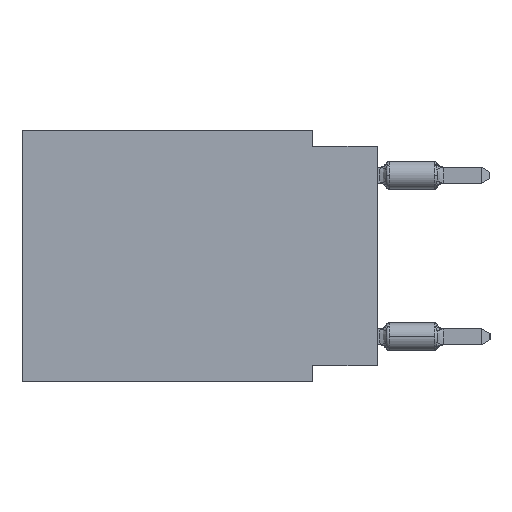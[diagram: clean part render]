
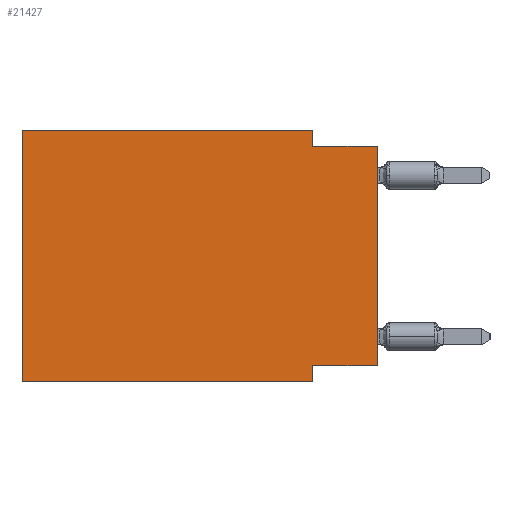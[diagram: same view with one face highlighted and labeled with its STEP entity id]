
A CAD part, left-side view. The second image highlights one B-rep face of the part: STEP entity #21427.
In plain terms, the highlighted planar face has unit normal (-1, 0, 0).
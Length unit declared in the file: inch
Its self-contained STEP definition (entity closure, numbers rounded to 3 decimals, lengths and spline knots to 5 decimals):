
#96 = CARTESIAN_POINT ( 'NONE',  ( 0., 0.55, 0. ) ) ;
#1198 = CARTESIAN_POINT ( 'NONE',  ( 0., 0.1, 0. ) ) ;
#1416 = DIRECTION ( 'NONE',  ( 0., 0., -1. ) ) ;
#1516 = EDGE_LOOP ( 'NONE', ( #18614, #11965, #40280, #30509, #34123, #24279, #11239, #11448 ) ) ;
#1558 = CARTESIAN_POINT ( 'NONE',  ( 0., 0.1, 0. ) ) ;
#2516 = EDGE_CURVE ( 'NONE', #9751, #14857, #4752, .T. ) ;
#2631 = EDGE_CURVE ( 'NONE', #19901, #14253, #5404, .T. ) ;
#2844 = VECTOR ( 'NONE', #1416, 39.37008 ) ;
#4245 = VERTEX_POINT ( 'NONE', #96 ) ;
#4752 = LINE ( 'NONE', #18272, #2844 ) ;
#5187 = VECTOR ( 'NONE', #41019, 39.37008 ) ;
#5231 = CARTESIAN_POINT ( 'NONE',  ( 0., 0.55, -0.39 ) ) ;
#5404 = LINE ( 'NONE', #19139, #32566 ) ;
#5408 = LINE ( 'NONE', #1198, #36933 ) ;
#8339 = DIRECTION ( 'NONE',  ( 0., -1., 0. ) ) ;
#9701 = CARTESIAN_POINT ( 'NONE',  ( 0., 0.1, -0.39 ) ) ;
#9704 = DIRECTION ( 'NONE',  ( 0., 1., 0. ) ) ;
#9751 = VERTEX_POINT ( 'NONE', #39318 ) ;
#9925 = CARTESIAN_POINT ( 'NONE',  ( 0., 0., -0.365 ) ) ;
#11239 = ORIENTED_EDGE ( 'NONE', *, *, #2516, .F. ) ;
#11354 = FACE_OUTER_BOUND ( 'NONE', #1516, .T. ) ;
#11448 = ORIENTED_EDGE ( 'NONE', *, *, #34178, .F. ) ;
#11965 = ORIENTED_EDGE ( 'NONE', *, *, #37853, .F. ) ;
#12773 = DIRECTION ( 'NONE',  ( 0., -1., 0. ) ) ;
#12815 = DIRECTION ( 'NONE',  ( 0., 0., -1. ) ) ;
#13987 = LINE ( 'NONE', #24176, #5187 ) ;
#14253 = VERTEX_POINT ( 'NONE', #35989 ) ;
#14857 = VERTEX_POINT ( 'NONE', #9701 ) ;
#17372 = VERTEX_POINT ( 'NONE', #1558 ) ;
#18272 = CARTESIAN_POINT ( 'NONE',  ( 0., 0.1, -0.39 ) ) ;
#18494 = DIRECTION ( 'NONE',  ( 0., 0., -1. ) ) ;
#18614 = ORIENTED_EDGE ( 'NONE', *, *, #2631, .T. ) ;
#18812 = CARTESIAN_POINT ( 'NONE',  ( 0., 0.55, 0. ) ) ;
#19139 = CARTESIAN_POINT ( 'NONE',  ( 0., 0., 0. ) ) ;
#19901 = VERTEX_POINT ( 'NONE', #39906 ) ;
#20064 = LINE ( 'NONE', #43772, #32785 ) ;
#20338 = VECTOR ( 'NONE', #9704, 39.37008 ) ;
#21427 = ADVANCED_FACE ( 'NONE', ( #11354 ), #26325, .F. ) ;
#24176 = CARTESIAN_POINT ( 'NONE',  ( 0., 0.55, 0. ) ) ;
#24279 = ORIENTED_EDGE ( 'NONE', *, *, #38174, .T. ) ;
#26143 = DIRECTION ( 'NONE',  ( 0., -1., 0. ) ) ;
#26325 = PLANE ( 'NONE',  #37262 ) ;
#30509 = ORIENTED_EDGE ( 'NONE', *, *, #43373, .F. ) ;
#30599 = VERTEX_POINT ( 'NONE', #30624 ) ;
#30624 = CARTESIAN_POINT ( 'NONE',  ( 0., 0.55, -0.39 ) ) ;
#31096 = EDGE_CURVE ( 'NONE', #30599, #4245, #13987, .T. ) ;
#32556 = DIRECTION ( 'NONE',  ( 1., 0., 0. ) ) ;
#32566 = VECTOR ( 'NONE', #43281, 39.37008 ) ;
#32785 = VECTOR ( 'NONE', #12773, 39.37008 ) ;
#33382 = VERTEX_POINT ( 'NONE', #33735 ) ;
#33735 = CARTESIAN_POINT ( 'NONE',  ( 0., 0.1, -0.025 ) ) ;
#34123 = ORIENTED_EDGE ( 'NONE', *, *, #31096, .F. ) ;
#34178 = EDGE_CURVE ( 'NONE', #19901, #9751, #40501, .T. ) ;
#35989 = CARTESIAN_POINT ( 'NONE',  ( 0., 0., -0.025 ) ) ;
#36933 = VECTOR ( 'NONE', #18494, 39.37008 ) ;
#37262 = AXIS2_PLACEMENT_3D ( 'NONE', #18812, #32556, #12815 ) ;
#37853 = EDGE_CURVE ( 'NONE', #33382, #14253, #42783, .T. ) ;
#38174 = EDGE_CURVE ( 'NONE', #30599, #14857, #38926, .T. ) ;
#38227 = VECTOR ( 'NONE', #26143, 39.37008 ) ;
#38926 = LINE ( 'NONE', #5231, #38961 ) ;
#38961 = VECTOR ( 'NONE', #8339, 39.37008 ) ;
#39318 = CARTESIAN_POINT ( 'NONE',  ( 0., 0.1, -0.365 ) ) ;
#39902 = CARTESIAN_POINT ( 'NONE',  ( 0., 0., -0.025 ) ) ;
#39906 = CARTESIAN_POINT ( 'NONE',  ( 0., 0., -0.365 ) ) ;
#40280 = ORIENTED_EDGE ( 'NONE', *, *, #42364, .F. ) ;
#40501 = LINE ( 'NONE', #9925, #20338 ) ;
#41019 = DIRECTION ( 'NONE',  ( 0., 0., 1. ) ) ;
#42364 = EDGE_CURVE ( 'NONE', #17372, #33382, #5408, .T. ) ;
#42783 = LINE ( 'NONE', #39902, #38227 ) ;
#43281 = DIRECTION ( 'NONE',  ( 0., 0., 1. ) ) ;
#43373 = EDGE_CURVE ( 'NONE', #4245, #17372, #20064, .T. ) ;
#43772 = CARTESIAN_POINT ( 'NONE',  ( 0., 0.55, 0. ) ) ;
